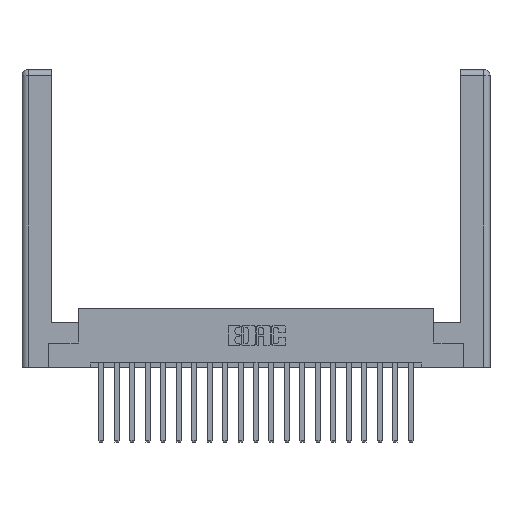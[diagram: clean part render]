
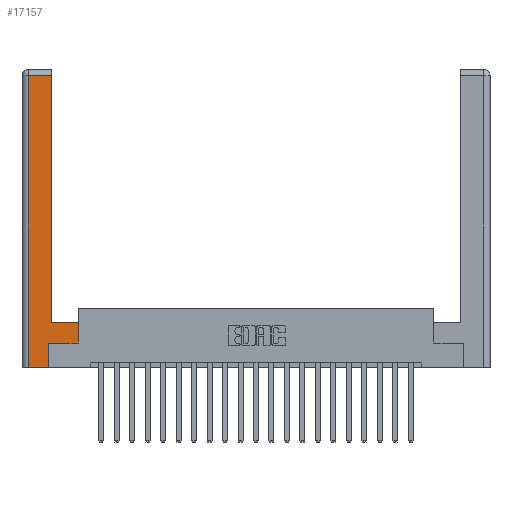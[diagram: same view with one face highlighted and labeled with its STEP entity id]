
A CAD part, top view. The second image highlights one B-rep face of the part: STEP entity #17157.
In plain terms, the highlighted planar face has unit normal (0, 0, 1).
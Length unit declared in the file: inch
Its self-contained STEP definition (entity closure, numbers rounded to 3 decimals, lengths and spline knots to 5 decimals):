
#141 = CARTESIAN_POINT ( 'NONE',  ( 0.0615, 0., 0. ) ) ;
#359 = FACE_OUTER_BOUND ( 'NONE', #10730, .T. ) ;
#579 = LINE ( 'NONE', #5719, #16927 ) ;
#1041 = CARTESIAN_POINT ( 'NONE',  ( 0.265, 0.245, 0. ) ) ;
#1134 = CARTESIAN_POINT ( 'NONE',  ( 0.0615, 2.94, 0. ) ) ;
#1176 = DIRECTION ( 'NONE',  ( 0., 1., 0. ) ) ;
#1804 = PLANE ( 'NONE',  #15883 ) ;
#1933 = LINE ( 'NONE', #1134, #20058 ) ;
#2213 = VERTEX_POINT ( 'NONE', #11313 ) ;
#2304 = VECTOR ( 'NONE', #17020, 39.37008 ) ;
#2856 = ORIENTED_EDGE ( 'NONE', *, *, #8383, .T. ) ;
#2962 = CARTESIAN_POINT ( 'NONE',  ( 0.265, 0., 0. ) ) ;
#3857 = EDGE_CURVE ( 'NONE', #10330, #19974, #18592, .T. ) ;
#4103 = VERTEX_POINT ( 'NONE', #9393 ) ;
#4365 = DIRECTION ( 'NONE',  ( 1., 0., 0. ) ) ;
#5474 = ORIENTED_EDGE ( 'NONE', *, *, #3857, .T. ) ;
#5719 = CARTESIAN_POINT ( 'NONE',  ( 0.295, 3., 0. ) ) ;
#6399 = DIRECTION ( 'NONE',  ( 0., 1., 0. ) ) ;
#7489 = EDGE_CURVE ( 'NONE', #4103, #11009, #1933, .T. ) ;
#7646 = DIRECTION ( 'NONE',  ( -1., 0., 0. ) ) ;
#7838 = VERTEX_POINT ( 'NONE', #10807 ) ;
#8383 = EDGE_CURVE ( 'NONE', #2213, #4103, #579, .T. ) ;
#8532 = VECTOR ( 'NONE', #14073, 39.37008 ) ;
#8584 = DIRECTION ( 'NONE',  ( -1., 0., 0. ) ) ;
#8663 = CARTESIAN_POINT ( 'NONE',  ( 0.565, 0.245, 0. ) ) ;
#9105 = LINE ( 'NONE', #18545, #16930 ) ;
#9393 = CARTESIAN_POINT ( 'NONE',  ( 0.295, 2.94, 0. ) ) ;
#9652 = EDGE_CURVE ( 'NONE', #7838, #10330, #15587, .T. ) ;
#10330 = VERTEX_POINT ( 'NONE', #8663 ) ;
#10416 = EDGE_CURVE ( 'NONE', #11009, #20361, #12133, .T. ) ;
#10730 = EDGE_LOOP ( 'NONE', ( #2856, #19813, #17267, #18045, #11621, #20379, #5474, #17948 ) ) ;
#10807 = CARTESIAN_POINT ( 'NONE',  ( 0.265, 0.245, 0. ) ) ;
#11009 = VERTEX_POINT ( 'NONE', #11455 ) ;
#11313 = CARTESIAN_POINT ( 'NONE',  ( 0.295, 0.45, 0. ) ) ;
#11455 = CARTESIAN_POINT ( 'NONE',  ( 0.0615, 2.94, 0. ) ) ;
#11456 = EDGE_CURVE ( 'NONE', #20361, #14503, #14226, .T. ) ;
#11615 = DIRECTION ( 'NONE',  ( 0., 0., -1. ) ) ;
#11621 = ORIENTED_EDGE ( 'NONE', *, *, #15708, .T. ) ;
#12133 = LINE ( 'NONE', #141, #2304 ) ;
#12768 = CARTESIAN_POINT ( 'NONE',  ( 0.265, 0., 0. ) ) ;
#13153 = CARTESIAN_POINT ( 'NONE',  ( 0.565, 0.45, 0. ) ) ;
#14073 = DIRECTION ( 'NONE',  ( 1., 0., 0. ) ) ;
#14226 = LINE ( 'NONE', #12768, #18610 ) ;
#14503 = VERTEX_POINT ( 'NONE', #2962 ) ;
#14690 = CARTESIAN_POINT ( 'NONE',  ( 0.565, 0.45, 0. ) ) ;
#15587 = LINE ( 'NONE', #18991, #8532 ) ;
#15708 = EDGE_CURVE ( 'NONE', #14503, #7838, #20325, .T. ) ;
#15841 = CARTESIAN_POINT ( 'NONE',  ( 0.0615, 0., 0. ) ) ;
#15883 = AXIS2_PLACEMENT_3D ( 'NONE', #16728, #11615, #16883 ) ;
#16728 = CARTESIAN_POINT ( 'NONE',  ( 0., 0., 0. ) ) ;
#16883 = DIRECTION ( 'NONE',  ( -1., 0., 0. ) ) ;
#16927 = VECTOR ( 'NONE', #17236, 39.37008 ) ;
#16930 = VECTOR ( 'NONE', #8584, 39.37008 ) ;
#17020 = DIRECTION ( 'NONE',  ( 0., -1., 0. ) ) ;
#17157 = ADVANCED_FACE ( 'NONE', ( #359 ), #1804, .F. ) ;
#17236 = DIRECTION ( 'NONE',  ( 0., 1., 0. ) ) ;
#17267 = ORIENTED_EDGE ( 'NONE', *, *, #10416, .T. ) ;
#17287 = VECTOR ( 'NONE', #6399, 39.37008 ) ;
#17948 = ORIENTED_EDGE ( 'NONE', *, *, #19713, .T. ) ;
#18045 = ORIENTED_EDGE ( 'NONE', *, *, #11456, .T. ) ;
#18295 = VECTOR ( 'NONE', #1176, 39.37008 ) ;
#18545 = CARTESIAN_POINT ( 'NONE',  ( 0.295, 0.45, 0. ) ) ;
#18592 = LINE ( 'NONE', #14690, #17287 ) ;
#18610 = VECTOR ( 'NONE', #4365, 39.37008 ) ;
#18991 = CARTESIAN_POINT ( 'NONE',  ( 0.565, 0.245, 0. ) ) ;
#19713 = EDGE_CURVE ( 'NONE', #19974, #2213, #9105, .T. ) ;
#19813 = ORIENTED_EDGE ( 'NONE', *, *, #7489, .T. ) ;
#19974 = VERTEX_POINT ( 'NONE', #13153 ) ;
#20058 = VECTOR ( 'NONE', #7646, 39.37008 ) ;
#20325 = LINE ( 'NONE', #1041, #18295 ) ;
#20361 = VERTEX_POINT ( 'NONE', #15841 ) ;
#20379 = ORIENTED_EDGE ( 'NONE', *, *, #9652, .T. ) ;
